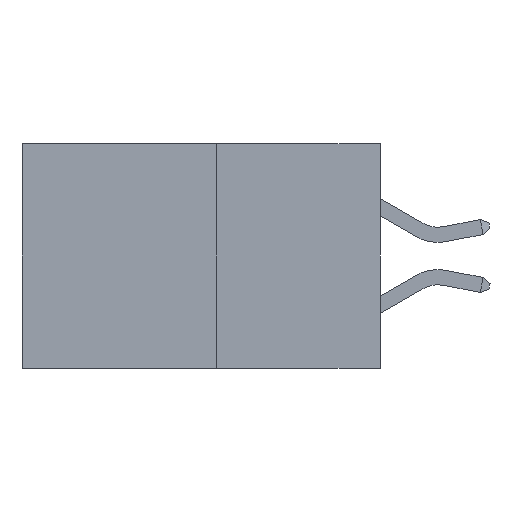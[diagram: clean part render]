
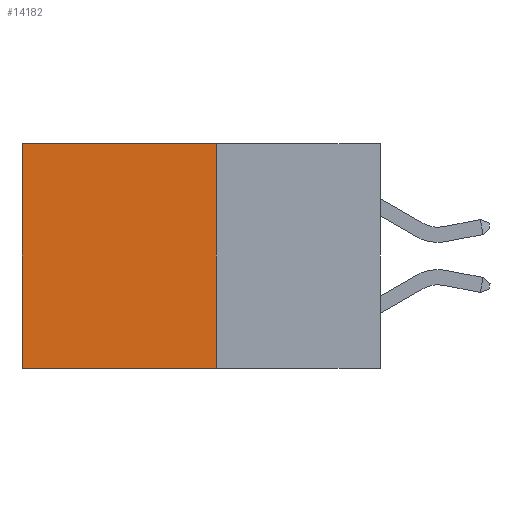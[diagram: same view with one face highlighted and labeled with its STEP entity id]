
A CAD part, left-side view. The second image highlights one B-rep face of the part: STEP entity #14182.
In plain terms, the highlighted planar face has unit normal (-1, 0, 0).
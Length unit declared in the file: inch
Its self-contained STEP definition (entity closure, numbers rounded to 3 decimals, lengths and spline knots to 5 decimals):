
#810 = VECTOR ( 'NONE', #12760, 39.37008 ) ;
#1180 = EDGE_LOOP ( 'NONE', ( #11358, #14693, #1967, #8769 ) ) ;
#1362 = CARTESIAN_POINT ( 'NONE',  ( 0.277, 0.59, -0.37 ) ) ;
#1967 = ORIENTED_EDGE ( 'NONE', *, *, #11819, .F. ) ;
#2256 = AXIS2_PLACEMENT_3D ( 'NONE', #9202, #13033, #5462 ) ;
#2738 = EDGE_CURVE ( 'NONE', #12495, #14865, #4717, .T. ) ;
#3638 = CARTESIAN_POINT ( 'NONE',  ( 0.277, 0.27, -0.37 ) ) ;
#3778 = VECTOR ( 'NONE', #4927, 39.37008 ) ;
#4188 = PLANE ( 'NONE',  #2256 ) ;
#4717 = LINE ( 'NONE', #5561, #810 ) ;
#4927 = DIRECTION ( 'NONE',  ( 0., 1., 0. ) ) ;
#5156 = VECTOR ( 'NONE', #10276, 39.37008 ) ;
#5462 = DIRECTION ( 'NONE',  ( 0., 0., -1. ) ) ;
#5561 = CARTESIAN_POINT ( 'NONE',  ( 0.277, 0.27, 0. ) ) ;
#6559 = DIRECTION ( 'NONE',  ( 0., 0., -1. ) ) ;
#7126 = LINE ( 'NONE', #3638, #3778 ) ;
#7564 = VERTEX_POINT ( 'NONE', #13768 ) ;
#7715 = CARTESIAN_POINT ( 'NONE',  ( 0.277, 0.27, 0. ) ) ;
#7736 = CARTESIAN_POINT ( 'NONE',  ( 0.277, 0.27, -0.37 ) ) ;
#7788 = VECTOR ( 'NONE', #6559, 39.37008 ) ;
#7945 = CARTESIAN_POINT ( 'NONE',  ( 0.277, 0.59, 0. ) ) ;
#8188 = VERTEX_POINT ( 'NONE', #12605 ) ;
#8481 = LINE ( 'NONE', #7736, #5156 ) ;
#8769 = ORIENTED_EDGE ( 'NONE', *, *, #2738, .T. ) ;
#9202 = CARTESIAN_POINT ( 'NONE',  ( 0.277, 0.27, -0.37 ) ) ;
#10276 = DIRECTION ( 'NONE',  ( 0., 0., -1. ) ) ;
#11269 = EDGE_CURVE ( 'NONE', #7564, #8188, #7126, .T. ) ;
#11358 = ORIENTED_EDGE ( 'NONE', *, *, #12545, .T. ) ;
#11568 = LINE ( 'NONE', #1362, #7788 ) ;
#11819 = EDGE_CURVE ( 'NONE', #12495, #7564, #8481, .T. ) ;
#12495 = VERTEX_POINT ( 'NONE', #7715 ) ;
#12545 = EDGE_CURVE ( 'NONE', #14865, #8188, #11568, .T. ) ;
#12605 = CARTESIAN_POINT ( 'NONE',  ( 0.277, 0.59, -0.37 ) ) ;
#12697 = FACE_OUTER_BOUND ( 'NONE', #1180, .T. ) ;
#12760 = DIRECTION ( 'NONE',  ( 0., 1., 0. ) ) ;
#13033 = DIRECTION ( 'NONE',  ( 1., 0., 0. ) ) ;
#13768 = CARTESIAN_POINT ( 'NONE',  ( 0.277, 0.27, -0.37 ) ) ;
#14182 = ADVANCED_FACE ( 'NONE', ( #12697 ), #4188, .F. ) ;
#14693 = ORIENTED_EDGE ( 'NONE', *, *, #11269, .F. ) ;
#14865 = VERTEX_POINT ( 'NONE', #7945 ) ;
